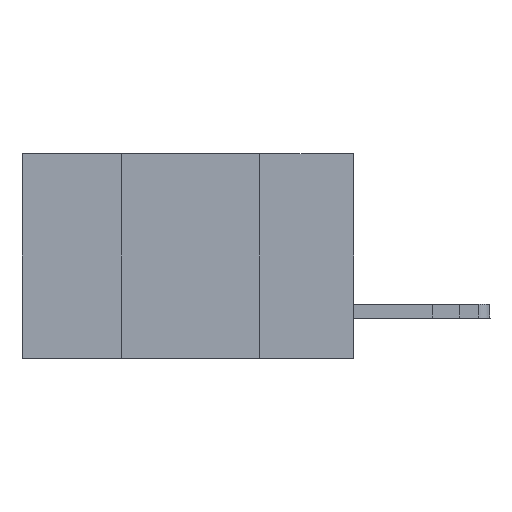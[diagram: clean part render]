
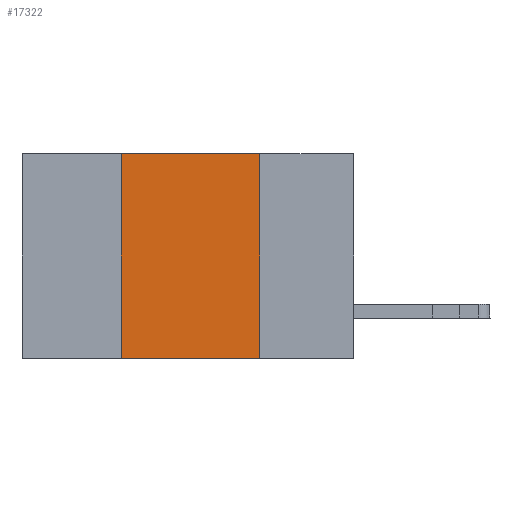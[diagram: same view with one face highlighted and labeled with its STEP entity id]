
A CAD part, left-side view. The second image highlights one B-rep face of the part: STEP entity #17322.
In plain terms, the highlighted planar face has unit normal (-1, 0, 0).
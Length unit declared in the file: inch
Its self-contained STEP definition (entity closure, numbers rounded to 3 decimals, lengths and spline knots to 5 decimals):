
#131 = EDGE_CURVE ( 'NONE', #13213, #1597, #697, .T. ) ;
#556 = CARTESIAN_POINT ( 'NONE',  ( 0., 0.42, 0. ) ) ;
#668 = CARTESIAN_POINT ( 'NONE',  ( 0., 0.17, -0.37 ) ) ;
#681 = ORIENTED_EDGE ( 'NONE', *, *, #14963, .F. ) ;
#697 = LINE ( 'NONE', #6746, #9190 ) ;
#1310 = DIRECTION ( 'NONE',  ( 0., -1., 0. ) ) ;
#1597 = VERTEX_POINT ( 'NONE', #556 ) ;
#2887 = EDGE_CURVE ( 'NONE', #13213, #6983, #3304, .T. ) ;
#3304 = LINE ( 'NONE', #6347, #20135 ) ;
#4202 = DIRECTION ( 'NONE',  ( 1., 0., 0. ) ) ;
#4921 = ORIENTED_EDGE ( 'NONE', *, *, #131, .F. ) ;
#6324 = DIRECTION ( 'NONE',  ( 0., -1., 0. ) ) ;
#6347 = CARTESIAN_POINT ( 'NONE',  ( 0., 0.6, -0.37 ) ) ;
#6746 = CARTESIAN_POINT ( 'NONE',  ( 0., 0.42, 0. ) ) ;
#6983 = VERTEX_POINT ( 'NONE', #668 ) ;
#7291 = PLANE ( 'NONE',  #7610 ) ;
#7445 = LINE ( 'NONE', #18662, #15939 ) ;
#7610 = AXIS2_PLACEMENT_3D ( 'NONE', #13747, #4202, #15333 ) ;
#8794 = DIRECTION ( 'NONE',  ( 0., 0., 1. ) ) ;
#9190 = VECTOR ( 'NONE', #8794, 39.37008 ) ;
#9584 = LINE ( 'NONE', #19967, #13817 ) ;
#9871 = EDGE_CURVE ( 'NONE', #16561, #6983, #9584, .T. ) ;
#10902 = CARTESIAN_POINT ( 'NONE',  ( 0., 0.42, -0.37 ) ) ;
#12906 = ORIENTED_EDGE ( 'NONE', *, *, #9871, .F. ) ;
#13213 = VERTEX_POINT ( 'NONE', #10902 ) ;
#13747 = CARTESIAN_POINT ( 'NONE',  ( 0., 0.6, 0. ) ) ;
#13817 = VECTOR ( 'NONE', #18426, 39.37008 ) ;
#14400 = EDGE_LOOP ( 'NONE', ( #12906, #681, #4921, #18585 ) ) ;
#14963 = EDGE_CURVE ( 'NONE', #1597, #16561, #7445, .T. ) ;
#15333 = DIRECTION ( 'NONE',  ( 0., 0., -1. ) ) ;
#15939 = VECTOR ( 'NONE', #1310, 39.37008 ) ;
#16505 = CARTESIAN_POINT ( 'NONE',  ( 0., 0.17, 0. ) ) ;
#16561 = VERTEX_POINT ( 'NONE', #16505 ) ;
#17322 = ADVANCED_FACE ( 'NONE', ( #19998 ), #7291, .F. ) ;
#18426 = DIRECTION ( 'NONE',  ( 0., 0., -1. ) ) ;
#18585 = ORIENTED_EDGE ( 'NONE', *, *, #2887, .T. ) ;
#18662 = CARTESIAN_POINT ( 'NONE',  ( 0., 0.6, 0. ) ) ;
#19967 = CARTESIAN_POINT ( 'NONE',  ( 0., 0.17, 0. ) ) ;
#19998 = FACE_OUTER_BOUND ( 'NONE', #14400, .T. ) ;
#20135 = VECTOR ( 'NONE', #6324, 39.37008 ) ;
